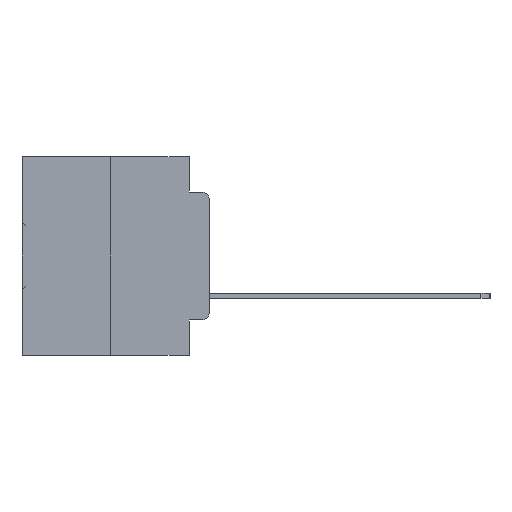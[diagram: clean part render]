
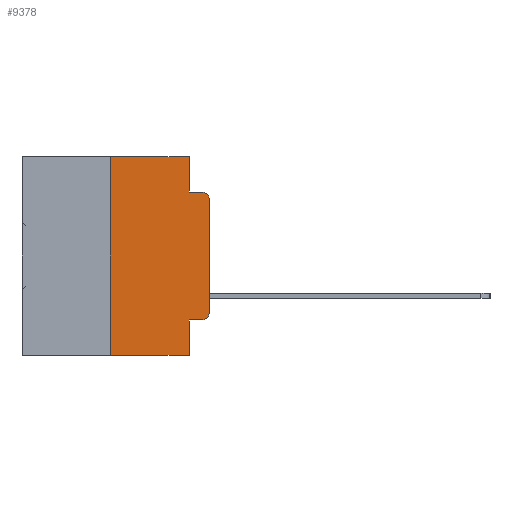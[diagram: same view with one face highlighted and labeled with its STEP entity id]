
A CAD part, left-side view. The second image highlights one B-rep face of the part: STEP entity #9378.
In plain terms, the highlighted planar face has unit normal (-1, 0, 0).
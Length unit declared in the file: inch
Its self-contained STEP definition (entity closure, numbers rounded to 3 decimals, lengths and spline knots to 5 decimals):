
#469 = CARTESIAN_POINT ( 'NONE',  ( 0., 0., 0. ) ) ;
#650 = ORIENTED_EDGE ( 'NONE', *, *, #12117, .F. ) ;
#2242 = EDGE_CURVE ( 'NONE', #16498, #31043, #20520, .T. ) ;
#3108 = VECTOR ( 'NONE', #31979, 39.37008 ) ;
#4127 = EDGE_CURVE ( 'NONE', #28331, #7937, #10547, .T. ) ;
#4196 = EDGE_CURVE ( 'NONE', #31043, #28331, #28848, .T. ) ;
#5034 = DIRECTION ( 'NONE',  ( 0., -1., 0. ) ) ;
#5411 = DIRECTION ( 'NONE',  ( -1., 0., 0. ) ) ;
#5439 = CARTESIAN_POINT ( 'NONE',  ( 0., 0.02, -0.4115 ) ) ;
#5531 = EDGE_LOOP ( 'NONE', ( #6308, #20962, #650, #28190, #8113, #10739, #7703, #9463, #14120, #34937 ) ) ;
#6232 = CARTESIAN_POINT ( 'NONE',  ( 0., 0.051, -0.4115 ) ) ;
#6308 = ORIENTED_EDGE ( 'NONE', *, *, #17613, .T. ) ;
#6415 = VERTEX_POINT ( 'NONE', #5439 ) ;
#6741 = VECTOR ( 'NONE', #13955, 39.37008 ) ;
#6753 = CARTESIAN_POINT ( 'NONE',  ( 0., 0.051, 0. ) ) ;
#7040 = VECTOR ( 'NONE', #7886, 39.37008 ) ;
#7246 = CARTESIAN_POINT ( 'NONE',  ( 0., 0.25, 0. ) ) ;
#7703 = ORIENTED_EDGE ( 'NONE', *, *, #19885, .T. ) ;
#7886 = DIRECTION ( 'NONE',  ( 0., -1., 0. ) ) ;
#7937 = VERTEX_POINT ( 'NONE', #28341 ) ;
#8113 = ORIENTED_EDGE ( 'NONE', *, *, #4196, .F. ) ;
#8484 = DIRECTION ( 'NONE',  ( 0., -1., 0. ) ) ;
#8644 = CARTESIAN_POINT ( 'NONE',  ( 0., 0.02, -0.1085 ) ) ;
#9378 = ADVANCED_FACE ( 'NONE', ( #18777 ), #27118, .F. ) ;
#9463 = ORIENTED_EDGE ( 'NONE', *, *, #32324, .F. ) ;
#10547 = LINE ( 'NONE', #18469, #3108 ) ;
#10739 = ORIENTED_EDGE ( 'NONE', *, *, #2242, .F. ) ;
#11180 = CARTESIAN_POINT ( 'NONE',  ( 0., 0.473, -0.5 ) ) ;
#11414 = DIRECTION ( 'NONE',  ( 0., 0., -1. ) ) ;
#11646 = DIRECTION ( 'NONE',  ( 0., 0., 1. ) ) ;
#12117 = EDGE_CURVE ( 'NONE', #7937, #20950, #22878, .T. ) ;
#13955 = DIRECTION ( 'NONE',  ( 0., -1., 0. ) ) ;
#14089 = VERTEX_POINT ( 'NONE', #19616 ) ;
#14120 = ORIENTED_EDGE ( 'NONE', *, *, #30512, .T. ) ;
#15767 = EDGE_CURVE ( 'NONE', #21344, #20950, #24703, .T. ) ;
#16064 = CARTESIAN_POINT ( 'NONE',  ( 0., 0.051, -0.4115 ) ) ;
#16291 = DIRECTION ( 'NONE',  ( 0., 0., -1. ) ) ;
#16498 = VERTEX_POINT ( 'NONE', #20449 ) ;
#17613 = EDGE_CURVE ( 'NONE', #14089, #21344, #22488, .T. ) ;
#17994 = AXIS2_PLACEMENT_3D ( 'NONE', #8644, #27726, #11414 ) ;
#18469 = CARTESIAN_POINT ( 'NONE',  ( 0., 0.051, 0. ) ) ;
#18707 = AXIS2_PLACEMENT_3D ( 'NONE', #21895, #5411, #24635 ) ;
#18777 = FACE_OUTER_BOUND ( 'NONE', #5531, .T. ) ;
#19616 = CARTESIAN_POINT ( 'NONE',  ( 0., 0., -0.3915 ) ) ;
#19885 = EDGE_CURVE ( 'NONE', #16498, #35428, #28570, .T. ) ;
#20449 = CARTESIAN_POINT ( 'NONE',  ( 0., 0.25, -0.5 ) ) ;
#20520 = LINE ( 'NONE', #28076, #34061 ) ;
#20950 = VERTEX_POINT ( 'NONE', #24715 ) ;
#20962 = ORIENTED_EDGE ( 'NONE', *, *, #15767, .T. ) ;
#21344 = VERTEX_POINT ( 'NONE', #29294 ) ;
#21895 = CARTESIAN_POINT ( 'NONE',  ( 0., 0.02, -0.3915 ) ) ;
#22488 = LINE ( 'NONE', #469, #28846 ) ;
#22510 = VECTOR ( 'NONE', #5034, 39.37008 ) ;
#22537 = DIRECTION ( 'NONE',  ( 0., 0., 1. ) ) ;
#22878 = LINE ( 'NONE', #24862, #23744 ) ;
#23133 = LINE ( 'NONE', #29717, #29477 ) ;
#23744 = VECTOR ( 'NONE', #8484, 39.37008 ) ;
#24635 = DIRECTION ( 'NONE',  ( 0., 0., -1. ) ) ;
#24703 = CIRCLE ( 'NONE', #17994, 0.02 ) ;
#24715 = CARTESIAN_POINT ( 'NONE',  ( 0., 0.02, -0.0885 ) ) ;
#24862 = CARTESIAN_POINT ( 'NONE',  ( 0., 0.051, -0.0885 ) ) ;
#26888 = VERTEX_POINT ( 'NONE', #6232 ) ;
#27022 = CARTESIAN_POINT ( 'NONE',  ( 0., 0.473, 0. ) ) ;
#27118 = PLANE ( 'NONE',  #31020 ) ;
#27726 = DIRECTION ( 'NONE',  ( -1., 0., 0. ) ) ;
#28076 = CARTESIAN_POINT ( 'NONE',  ( 0., 0.25, 0. ) ) ;
#28190 = ORIENTED_EDGE ( 'NONE', *, *, #4127, .F. ) ;
#28331 = VERTEX_POINT ( 'NONE', #6753 ) ;
#28341 = CARTESIAN_POINT ( 'NONE',  ( 0., 0.051, -0.0885 ) ) ;
#28570 = LINE ( 'NONE', #11180, #6741 ) ;
#28704 = EDGE_CURVE ( 'NONE', #6415, #14089, #31066, .T. ) ;
#28846 = VECTOR ( 'NONE', #22537, 39.37008 ) ;
#28848 = LINE ( 'NONE', #27022, #7040 ) ;
#29294 = CARTESIAN_POINT ( 'NONE',  ( 0., 0., -0.1085 ) ) ;
#29442 = CARTESIAN_POINT ( 'NONE',  ( 0., 0.051, -0.5 ) ) ;
#29477 = VECTOR ( 'NONE', #35130, 39.37008 ) ;
#29693 = LINE ( 'NONE', #16064, #22510 ) ;
#29717 = CARTESIAN_POINT ( 'NONE',  ( 0., 0.051, 0. ) ) ;
#29802 = CARTESIAN_POINT ( 'NONE',  ( 0., 0.473, 0. ) ) ;
#30512 = EDGE_CURVE ( 'NONE', #26888, #6415, #29693, .T. ) ;
#31020 = AXIS2_PLACEMENT_3D ( 'NONE', #29802, #32523, #16291 ) ;
#31043 = VERTEX_POINT ( 'NONE', #7246 ) ;
#31066 = CIRCLE ( 'NONE', #18707, 0.02 ) ;
#31979 = DIRECTION ( 'NONE',  ( 0., 0., -1. ) ) ;
#32324 = EDGE_CURVE ( 'NONE', #26888, #35428, #23133, .T. ) ;
#32523 = DIRECTION ( 'NONE',  ( 1., 0., 0. ) ) ;
#34061 = VECTOR ( 'NONE', #11646, 39.37008 ) ;
#34937 = ORIENTED_EDGE ( 'NONE', *, *, #28704, .T. ) ;
#35130 = DIRECTION ( 'NONE',  ( 0., 0., -1. ) ) ;
#35428 = VERTEX_POINT ( 'NONE', #29442 ) ;
